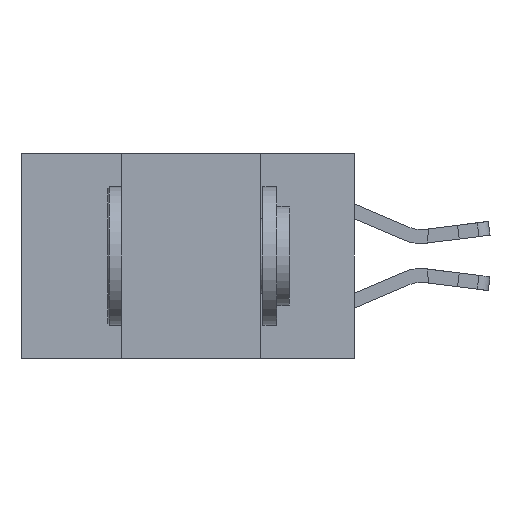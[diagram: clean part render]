
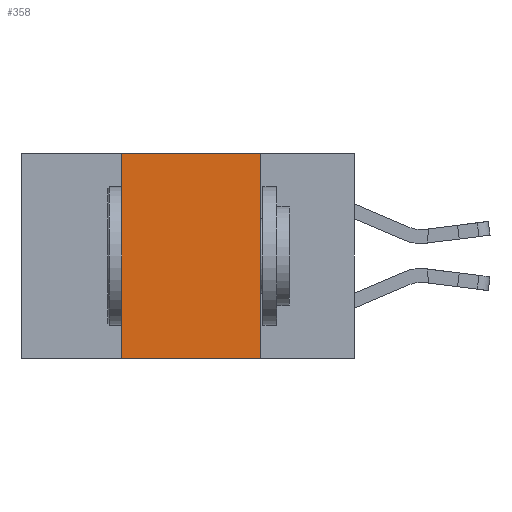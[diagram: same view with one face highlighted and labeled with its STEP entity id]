
A CAD part, left-side view. The second image highlights one B-rep face of the part: STEP entity #358.
In plain terms, the highlighted planar face has unit normal (-1, 0, 0).
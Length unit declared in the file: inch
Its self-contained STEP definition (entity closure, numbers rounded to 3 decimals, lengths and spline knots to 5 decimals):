
#113 = CARTESIAN_POINT ( 'NONE',  ( 0., 0.6, 0. ) ) ;
#358 = ADVANCED_FACE ( 'NONE', ( #3003 ), #11515, .F. ) ;
#710 = CARTESIAN_POINT ( 'NONE',  ( 0., 0.42, -0.37 ) ) ;
#1012 = VERTEX_POINT ( 'NONE', #11481 ) ;
#1951 = CARTESIAN_POINT ( 'NONE',  ( 0., 0.6, 0. ) ) ;
#1973 = ORIENTED_EDGE ( 'NONE', *, *, #2670, .F. ) ;
#2027 = DIRECTION ( 'NONE',  ( 1., 0., 0. ) ) ;
#2670 = EDGE_CURVE ( 'NONE', #1012, #11279, #11145, .T. ) ;
#3003 = FACE_OUTER_BOUND ( 'NONE', #4281, .T. ) ;
#3396 = DIRECTION ( 'NONE',  ( 0., -1., 0. ) ) ;
#4281 = EDGE_LOOP ( 'NONE', ( #1973, #7649, #7776, #11268 ) ) ;
#4678 = VERTEX_POINT ( 'NONE', #9384 ) ;
#5146 = VECTOR ( 'NONE', #3396, 39.37008 ) ;
#5429 = LINE ( 'NONE', #113, #5146 ) ;
#5854 = EDGE_CURVE ( 'NONE', #4678, #1012, #5429, .T. ) ;
#6204 = DIRECTION ( 'NONE',  ( 0., 0., -1. ) ) ;
#6512 = CARTESIAN_POINT ( 'NONE',  ( 0., 0.6, -0.37 ) ) ;
#7439 = CARTESIAN_POINT ( 'NONE',  ( 0., 0.17, -0.37 ) ) ;
#7649 = ORIENTED_EDGE ( 'NONE', *, *, #5854, .F. ) ;
#7776 = ORIENTED_EDGE ( 'NONE', *, *, #10448, .F. ) ;
#8194 = DIRECTION ( 'NONE',  ( 0., 0., 1. ) ) ;
#9384 = CARTESIAN_POINT ( 'NONE',  ( 0., 0.42, 0. ) ) ;
#9639 = VECTOR ( 'NONE', #8194, 39.37008 ) ;
#9690 = VECTOR ( 'NONE', #10694, 39.37008 ) ;
#10165 = CARTESIAN_POINT ( 'NONE',  ( 0., 0.17, -0.37 ) ) ;
#10351 = VERTEX_POINT ( 'NONE', #710 ) ;
#10448 = EDGE_CURVE ( 'NONE', #10351, #4678, #11330, .T. ) ;
#10620 = LINE ( 'NONE', #6512, #9690 ) ;
#10694 = DIRECTION ( 'NONE',  ( 0., -1., 0. ) ) ;
#11145 = LINE ( 'NONE', #10165, #12422 ) ;
#11268 = ORIENTED_EDGE ( 'NONE', *, *, #13091, .T. ) ;
#11279 = VERTEX_POINT ( 'NONE', #7439 ) ;
#11330 = LINE ( 'NONE', #13470, #9639 ) ;
#11481 = CARTESIAN_POINT ( 'NONE',  ( 0., 0.17, 0. ) ) ;
#11515 = PLANE ( 'NONE',  #12386 ) ;
#12183 = DIRECTION ( 'NONE',  ( 0., 0., -1. ) ) ;
#12386 = AXIS2_PLACEMENT_3D ( 'NONE', #1951, #2027, #6204 ) ;
#12422 = VECTOR ( 'NONE', #12183, 39.37008 ) ;
#13091 = EDGE_CURVE ( 'NONE', #10351, #11279, #10620, .T. ) ;
#13470 = CARTESIAN_POINT ( 'NONE',  ( 0., 0.42, -0.37 ) ) ;
